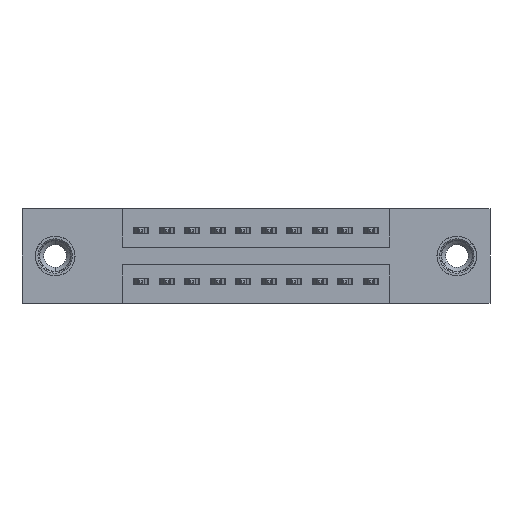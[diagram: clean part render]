
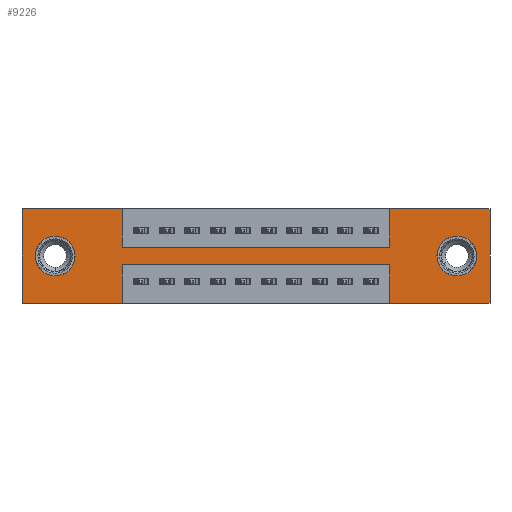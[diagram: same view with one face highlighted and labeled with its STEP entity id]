
A CAD part, front view. The second image highlights one B-rep face of the part: STEP entity #9226.
In plain terms, the highlighted planar face has unit normal (0, -1, 0).
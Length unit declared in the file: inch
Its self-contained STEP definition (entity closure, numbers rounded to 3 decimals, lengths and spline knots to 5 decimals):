
#96 = VECTOR ( 'NONE', #6791, 39.37008 ) ;
#114 = VERTEX_POINT ( 'NONE', #4557 ) ;
#384 = VERTEX_POINT ( 'NONE', #11024 ) ;
#857 = CARTESIAN_POINT ( 'NONE',  ( 1.835, 0., -0.37 ) ) ;
#906 = DIRECTION ( 'NONE',  ( -1., 0., 0. ) ) ;
#921 = VERTEX_POINT ( 'NONE', #7659 ) ;
#1037 = DIRECTION ( 'NONE',  ( 0., 1., 0. ) ) ;
#1117 = ORIENTED_EDGE ( 'NONE', *, *, #5726, .T. ) ;
#1210 = VERTEX_POINT ( 'NONE', #6740 ) ;
#1260 = VECTOR ( 'NONE', #10769, 39.37008 ) ;
#1335 = DIRECTION ( 'NONE',  ( 0., 1., 0. ) ) ;
#1416 = CARTESIAN_POINT ( 'NONE',  ( 0.3925, 0., 0. ) ) ;
#1462 = ORIENTED_EDGE ( 'NONE', *, *, #7943, .F. ) ;
#1504 = EDGE_CURVE ( 'NONE', #12181, #9555, #6871, .T. ) ;
#1562 = PLANE ( 'NONE',  #5815 ) ;
#1608 = LINE ( 'NONE', #3528, #4752 ) ;
#1742 = DIRECTION ( 'NONE',  ( 0., 1., 0. ) ) ;
#1750 = EDGE_CURVE ( 'NONE', #6777, #2295, #6703, .T. ) ;
#1946 = DIRECTION ( 'NONE',  ( -1., 0., 0. ) ) ;
#2018 = VECTOR ( 'NONE', #3727, 39.37008 ) ;
#2041 = CARTESIAN_POINT ( 'NONE',  ( 1.4425, 0., -0.15 ) ) ;
#2202 = LINE ( 'NONE', #4024, #13064 ) ;
#2295 = VERTEX_POINT ( 'NONE', #2317 ) ;
#2317 = CARTESIAN_POINT ( 'NONE',  ( 0.13, 0., -0.263 ) ) ;
#2357 = DIRECTION ( 'NONE',  ( 0., 0., 1. ) ) ;
#2632 = CARTESIAN_POINT ( 'NONE',  ( 0., 0., -0.37 ) ) ;
#2647 = CARTESIAN_POINT ( 'NONE',  ( 0.3925, 0., -0.37 ) ) ;
#2841 = CARTESIAN_POINT ( 'NONE',  ( 0., 0., 0. ) ) ;
#2878 = CARTESIAN_POINT ( 'NONE',  ( 1.705, 0., -0.263 ) ) ;
#2944 = CIRCLE ( 'NONE', #10821, 0.078 ) ;
#2972 = DIRECTION ( 'NONE',  ( 0., 0., -1. ) ) ;
#3052 = CIRCLE ( 'NONE', #8580, 0.078 ) ;
#3438 = EDGE_LOOP ( 'NONE', ( #3620, #1117 ) ) ;
#3449 = LINE ( 'NONE', #8470, #5626 ) ;
#3489 = EDGE_CURVE ( 'NONE', #384, #6060, #10539, .T. ) ;
#3528 = CARTESIAN_POINT ( 'NONE',  ( 1.4425, 0., -0.37 ) ) ;
#3620 = ORIENTED_EDGE ( 'NONE', *, *, #1750, .T. ) ;
#3624 = CARTESIAN_POINT ( 'NONE',  ( 0., 0., 0. ) ) ;
#3727 = DIRECTION ( 'NONE',  ( 1., 0., 0. ) ) ;
#3949 = ORIENTED_EDGE ( 'NONE', *, *, #10464, .F. ) ;
#4024 = CARTESIAN_POINT ( 'NONE',  ( 0.3925, 0., -0.37 ) ) ;
#4107 = EDGE_LOOP ( 'NONE', ( #3949, #12071, #1462, #4284, #9745, #12387, #4619, #10043, #7766, #10346, #8074, #13323 ) ) ;
#4144 = CARTESIAN_POINT ( 'NONE',  ( 0.3925, 0., -0.22 ) ) ;
#4284 = ORIENTED_EDGE ( 'NONE', *, *, #13333, .F. ) ;
#4299 = DIRECTION ( 'NONE',  ( 0., 0., 1. ) ) ;
#4381 = FACE_BOUND ( 'NONE', #3438, .T. ) ;
#4484 = CARTESIAN_POINT ( 'NONE',  ( 1.4425, 0., 0. ) ) ;
#4557 = CARTESIAN_POINT ( 'NONE',  ( 1.835, 0., 0. ) ) ;
#4619 = ORIENTED_EDGE ( 'NONE', *, *, #9057, .F. ) ;
#4684 = DIRECTION ( 'NONE',  ( 0., 1., 0. ) ) ;
#4737 = VERTEX_POINT ( 'NONE', #4144 ) ;
#4752 = VECTOR ( 'NONE', #10676, 39.37008 ) ;
#4755 = DIRECTION ( 'NONE',  ( 0., -1., 0. ) ) ;
#5094 = LINE ( 'NONE', #11301, #7581 ) ;
#5137 = CARTESIAN_POINT ( 'NONE',  ( 0.3925, 0., -0.22 ) ) ;
#5250 = EDGE_CURVE ( 'NONE', #1210, #114, #11125, .T. ) ;
#5468 = LINE ( 'NONE', #5137, #10195 ) ;
#5626 = VECTOR ( 'NONE', #4299, 39.37008 ) ;
#5726 = EDGE_CURVE ( 'NONE', #2295, #6777, #2944, .T. ) ;
#5736 = CARTESIAN_POINT ( 'NONE',  ( 1.835, 0., 0. ) ) ;
#5803 = LINE ( 'NONE', #5736, #96 ) ;
#5815 = AXIS2_PLACEMENT_3D ( 'NONE', #2632, #4755, #11859 ) ;
#6027 = EDGE_CURVE ( 'NONE', #6425, #4737, #5468, .T. ) ;
#6060 = VERTEX_POINT ( 'NONE', #2041 ) ;
#6104 = EDGE_CURVE ( 'NONE', #8198, #13207, #6281, .T. ) ;
#6149 = EDGE_CURVE ( 'NONE', #9555, #12940, #3449, .T. ) ;
#6199 = CARTESIAN_POINT ( 'NONE',  ( 0., 0., 0. ) ) ;
#6224 = CARTESIAN_POINT ( 'NONE',  ( 0., 0., -0.37 ) ) ;
#6255 = LINE ( 'NONE', #3624, #1260 ) ;
#6281 = CIRCLE ( 'NONE', #11926, 0.078 ) ;
#6375 = CARTESIAN_POINT ( 'NONE',  ( 1.4425, 0., -0.37 ) ) ;
#6425 = VERTEX_POINT ( 'NONE', #11779 ) ;
#6703 = CIRCLE ( 'NONE', #13141, 0.078 ) ;
#6740 = CARTESIAN_POINT ( 'NONE',  ( 1.4425, 0., 0. ) ) ;
#6777 = VERTEX_POINT ( 'NONE', #10518 ) ;
#6791 = DIRECTION ( 'NONE',  ( 0., 0., -1. ) ) ;
#6871 = LINE ( 'NONE', #6224, #11864 ) ;
#6923 = EDGE_CURVE ( 'NONE', #114, #10476, #5803, .T. ) ;
#7180 = CARTESIAN_POINT ( 'NONE',  ( 1.705, 0., -0.107 ) ) ;
#7400 = CARTESIAN_POINT ( 'NONE',  ( 1.705, 0., -0.185 ) ) ;
#7581 = VECTOR ( 'NONE', #12293, 39.37008 ) ;
#7659 = CARTESIAN_POINT ( 'NONE',  ( 0.3925, 0., 0. ) ) ;
#7688 = CARTESIAN_POINT ( 'NONE',  ( 0.13, 0., -0.185 ) ) ;
#7766 = ORIENTED_EDGE ( 'NONE', *, *, #9127, .F. ) ;
#7943 = EDGE_CURVE ( 'NONE', #9597, #6425, #1608, .T. ) ;
#8002 = EDGE_CURVE ( 'NONE', #12940, #921, #6255, .T. ) ;
#8064 = CARTESIAN_POINT ( 'NONE',  ( 1.705, 0., -0.185 ) ) ;
#8074 = ORIENTED_EDGE ( 'NONE', *, *, #6149, .F. ) ;
#8198 = VERTEX_POINT ( 'NONE', #2878 ) ;
#8426 = DIRECTION ( 'NONE',  ( 0., 0., -1. ) ) ;
#8470 = CARTESIAN_POINT ( 'NONE',  ( 0., 0., 0. ) ) ;
#8580 = AXIS2_PLACEMENT_3D ( 'NONE', #8064, #1742, #9035 ) ;
#8694 = DIRECTION ( 'NONE',  ( 0., 0., 1. ) ) ;
#8843 = ORIENTED_EDGE ( 'NONE', *, *, #9349, .T. ) ;
#9035 = DIRECTION ( 'NONE',  ( 0., 0., -1. ) ) ;
#9057 = EDGE_CURVE ( 'NONE', #6060, #1210, #9390, .T. ) ;
#9073 = VECTOR ( 'NONE', #2357, 39.37008 ) ;
#9127 = EDGE_CURVE ( 'NONE', #921, #384, #11402, .T. ) ;
#9131 = EDGE_LOOP ( 'NONE', ( #8843, #11467 ) ) ;
#9226 = ADVANCED_FACE ( 'NONE', ( #9832, #4381, #12484 ), #1562, .T. ) ;
#9349 = EDGE_CURVE ( 'NONE', #13207, #8198, #3052, .T. ) ;
#9390 = LINE ( 'NONE', #4484, #9073 ) ;
#9555 = VERTEX_POINT ( 'NONE', #13325 ) ;
#9597 = VERTEX_POINT ( 'NONE', #6375 ) ;
#9745 = ORIENTED_EDGE ( 'NONE', *, *, #6923, .F. ) ;
#9832 = FACE_BOUND ( 'NONE', #9131, .T. ) ;
#10043 = ORIENTED_EDGE ( 'NONE', *, *, #3489, .F. ) ;
#10195 = VECTOR ( 'NONE', #1946, 39.37008 ) ;
#10346 = ORIENTED_EDGE ( 'NONE', *, *, #8002, .F. ) ;
#10464 = EDGE_CURVE ( 'NONE', #4737, #12181, #2202, .T. ) ;
#10476 = VERTEX_POINT ( 'NONE', #857 ) ;
#10518 = CARTESIAN_POINT ( 'NONE',  ( 0.13, 0., -0.107 ) ) ;
#10539 = LINE ( 'NONE', #11403, #2018 ) ;
#10676 = DIRECTION ( 'NONE',  ( 0., 0., 1. ) ) ;
#10695 = DIRECTION ( 'NONE',  ( 0., 0., -1. ) ) ;
#10745 = VECTOR ( 'NONE', #10695, 39.37008 ) ;
#10758 = CARTESIAN_POINT ( 'NONE',  ( 0.13, 0., -0.185 ) ) ;
#10769 = DIRECTION ( 'NONE',  ( 1., 0., 0. ) ) ;
#10810 = VECTOR ( 'NONE', #12047, 39.37008 ) ;
#10821 = AXIS2_PLACEMENT_3D ( 'NONE', #10758, #4684, #11796 ) ;
#11024 = CARTESIAN_POINT ( 'NONE',  ( 0.3925, 0., -0.15 ) ) ;
#11125 = LINE ( 'NONE', #2841, #10810 ) ;
#11301 = CARTESIAN_POINT ( 'NONE',  ( 0., 0., -0.37 ) ) ;
#11402 = LINE ( 'NONE', #1416, #10745 ) ;
#11403 = CARTESIAN_POINT ( 'NONE',  ( 0.3925, 0., -0.15 ) ) ;
#11467 = ORIENTED_EDGE ( 'NONE', *, *, #6104, .T. ) ;
#11779 = CARTESIAN_POINT ( 'NONE',  ( 1.4425, 0., -0.22 ) ) ;
#11796 = DIRECTION ( 'NONE',  ( 0., 0., 1. ) ) ;
#11859 = DIRECTION ( 'NONE',  ( 0., 0., -1. ) ) ;
#11864 = VECTOR ( 'NONE', #906, 39.37008 ) ;
#11926 = AXIS2_PLACEMENT_3D ( 'NONE', #7400, #1037, #8426 ) ;
#12047 = DIRECTION ( 'NONE',  ( 1., 0., 0. ) ) ;
#12071 = ORIENTED_EDGE ( 'NONE', *, *, #6027, .F. ) ;
#12181 = VERTEX_POINT ( 'NONE', #2647 ) ;
#12293 = DIRECTION ( 'NONE',  ( -1., 0., 0. ) ) ;
#12387 = ORIENTED_EDGE ( 'NONE', *, *, #5250, .F. ) ;
#12484 = FACE_OUTER_BOUND ( 'NONE', #4107, .T. ) ;
#12940 = VERTEX_POINT ( 'NONE', #6199 ) ;
#13064 = VECTOR ( 'NONE', #2972, 39.37008 ) ;
#13141 = AXIS2_PLACEMENT_3D ( 'NONE', #7688, #1335, #8694 ) ;
#13207 = VERTEX_POINT ( 'NONE', #7180 ) ;
#13323 = ORIENTED_EDGE ( 'NONE', *, *, #1504, .F. ) ;
#13325 = CARTESIAN_POINT ( 'NONE',  ( 0., 0., -0.37 ) ) ;
#13333 = EDGE_CURVE ( 'NONE', #10476, #9597, #5094, .T. ) ;
